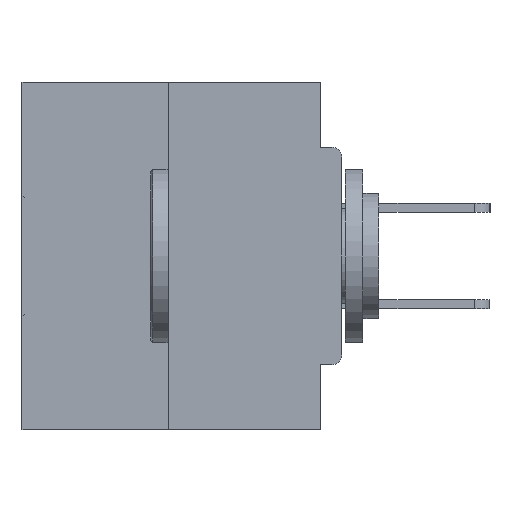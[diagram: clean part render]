
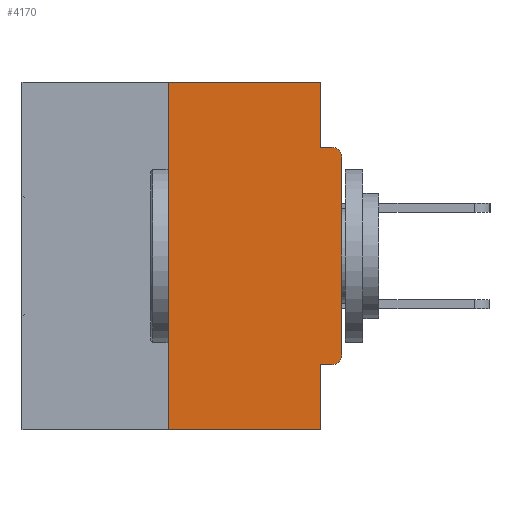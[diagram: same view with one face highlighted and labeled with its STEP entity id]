
A CAD part, left-side view. The second image highlights one B-rep face of the part: STEP entity #4170.
In plain terms, the highlighted planar face has unit normal (-1, 0, 0).
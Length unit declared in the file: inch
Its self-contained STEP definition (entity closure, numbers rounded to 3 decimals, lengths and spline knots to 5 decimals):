
#173 = DIRECTION ( 'NONE',  ( 0., -1., 0. ) ) ;
#609 = VERTEX_POINT ( 'NONE', #1921 ) ;
#1921 = CARTESIAN_POINT ( 'NONE',  ( 0., 0.25, -0.5 ) ) ;
#2100 = EDGE_CURVE ( 'NONE', #4146, #41468, #22063, .T. ) ;
#2630 = CARTESIAN_POINT ( 'NONE',  ( 0., 0.46, 0. ) ) ;
#4146 = VERTEX_POINT ( 'NONE', #24098 ) ;
#4170 = ADVANCED_FACE ( 'NONE', ( #25506 ), #5548, .F. ) ;
#4461 = CIRCLE ( 'NONE', #42442, 0.015 ) ;
#4488 = CARTESIAN_POINT ( 'NONE',  ( 0., 0.015, -0.4065 ) ) ;
#5046 = EDGE_CURVE ( 'NONE', #8070, #19093, #11988, .T. ) ;
#5341 = ORIENTED_EDGE ( 'NONE', *, *, #41812, .T. ) ;
#5405 = CARTESIAN_POINT ( 'NONE',  ( 0., 0.25, 0. ) ) ;
#5548 = PLANE ( 'NONE',  #42159 ) ;
#6233 = CARTESIAN_POINT ( 'NONE',  ( 0., 0.031, -0.5 ) ) ;
#6565 = CARTESIAN_POINT ( 'NONE',  ( 0., 0., -0.4065 ) ) ;
#6663 = VERTEX_POINT ( 'NONE', #5405 ) ;
#7348 = VECTOR ( 'NONE', #12847, 39.37008 ) ;
#8070 = VERTEX_POINT ( 'NONE', #35930 ) ;
#8725 = CARTESIAN_POINT ( 'NONE',  ( 0., 0.25, 0. ) ) ;
#8738 = VECTOR ( 'NONE', #18216, 39.37008 ) ;
#8857 = DIRECTION ( 'NONE',  ( 1., 0., 0. ) ) ;
#9143 = DIRECTION ( 'NONE',  ( 0., 0., -1. ) ) ;
#9898 = CARTESIAN_POINT ( 'NONE',  ( 0., 0., 0. ) ) ;
#10563 = VECTOR ( 'NONE', #173, 39.37008 ) ;
#11882 = LINE ( 'NONE', #35263, #31456 ) ;
#11988 = LINE ( 'NONE', #9898, #38200 ) ;
#12035 = VECTOR ( 'NONE', #12253, 39.37008 ) ;
#12110 = CARTESIAN_POINT ( 'NONE',  ( 0., 0.46, 0. ) ) ;
#12253 = DIRECTION ( 'NONE',  ( 0., -1., 0. ) ) ;
#12656 = VECTOR ( 'NONE', #31747, 39.37008 ) ;
#12847 = DIRECTION ( 'NONE',  ( 0., 1., 0. ) ) ;
#12949 = LINE ( 'NONE', #8725, #41744 ) ;
#14905 = EDGE_CURVE ( 'NONE', #6663, #24951, #20804, .T. ) ;
#15072 = ORIENTED_EDGE ( 'NONE', *, *, #33268, .T. ) ;
#15228 = LINE ( 'NONE', #31597, #12656 ) ;
#17316 = EDGE_CURVE ( 'NONE', #26795, #24085, #11882, .T. ) ;
#17340 = DIRECTION ( 'NONE',  ( -1., 0., 0. ) ) ;
#18037 = DIRECTION ( 'NONE',  ( 0., 0., -1. ) ) ;
#18216 = DIRECTION ( 'NONE',  ( 0., 0., -1. ) ) ;
#19093 = VERTEX_POINT ( 'NONE', #20516 ) ;
#20035 = EDGE_CURVE ( 'NONE', #609, #6663, #12949, .T. ) ;
#20224 = DIRECTION ( 'NONE',  ( 0., 0., 1. ) ) ;
#20516 = CARTESIAN_POINT ( 'NONE',  ( 0., 0., -0.1085 ) ) ;
#20804 = LINE ( 'NONE', #12110, #12035 ) ;
#21762 = AXIS2_PLACEMENT_3D ( 'NONE', #21901, #25218, #18037 ) ;
#21901 = CARTESIAN_POINT ( 'NONE',  ( 0., 0.015, -0.3915 ) ) ;
#22063 = LINE ( 'NONE', #41600, #8738 ) ;
#23034 = CARTESIAN_POINT ( 'NONE',  ( 0., 0.46, -0.5 ) ) ;
#23583 = CIRCLE ( 'NONE', #21762, 0.015 ) ;
#23715 = ORIENTED_EDGE ( 'NONE', *, *, #39460, .F. ) ;
#23766 = ORIENTED_EDGE ( 'NONE', *, *, #20035, .F. ) ;
#24085 = VERTEX_POINT ( 'NONE', #34598 ) ;
#24098 = CARTESIAN_POINT ( 'NONE',  ( 0., 0.031, -0.4065 ) ) ;
#24951 = VERTEX_POINT ( 'NONE', #33543 ) ;
#25218 = DIRECTION ( 'NONE',  ( -1., 0., 0. ) ) ;
#25506 = FACE_OUTER_BOUND ( 'NONE', #36485, .T. ) ;
#25969 = LINE ( 'NONE', #23034, #10563 ) ;
#26795 = VERTEX_POINT ( 'NONE', #27788 ) ;
#27027 = EDGE_CURVE ( 'NONE', #24951, #26795, #15228, .T. ) ;
#27199 = ORIENTED_EDGE ( 'NONE', *, *, #27027, .F. ) ;
#27788 = CARTESIAN_POINT ( 'NONE',  ( 0., 0.031, -0.0935 ) ) ;
#31456 = VECTOR ( 'NONE', #41605, 39.37008 ) ;
#31597 = CARTESIAN_POINT ( 'NONE',  ( 0., 0.031, 0. ) ) ;
#31747 = DIRECTION ( 'NONE',  ( 0., 0., -1. ) ) ;
#31844 = DIRECTION ( 'NONE',  ( 0., 0., 1. ) ) ;
#31912 = ORIENTED_EDGE ( 'NONE', *, *, #5046, .T. ) ;
#32146 = ORIENTED_EDGE ( 'NONE', *, *, #2100, .F. ) ;
#33109 = EDGE_CURVE ( 'NONE', #609, #41468, #25969, .T. ) ;
#33268 = EDGE_CURVE ( 'NONE', #19093, #24085, #4461, .T. ) ;
#33543 = CARTESIAN_POINT ( 'NONE',  ( 0., 0.031, 0. ) ) ;
#34019 = CARTESIAN_POINT ( 'NONE',  ( 0., 0.015, -0.1085 ) ) ;
#34598 = CARTESIAN_POINT ( 'NONE',  ( 0., 0.015, -0.0935 ) ) ;
#35263 = CARTESIAN_POINT ( 'NONE',  ( 0., 0., -0.0935 ) ) ;
#35503 = DIRECTION ( 'NONE',  ( 0., 0., -1. ) ) ;
#35930 = CARTESIAN_POINT ( 'NONE',  ( 0., 0., -0.3915 ) ) ;
#36485 = EDGE_LOOP ( 'NONE', ( #39961, #23766, #39555, #32146, #23715, #5341, #31912, #15072, #40087, #27199 ) ) ;
#38178 = VERTEX_POINT ( 'NONE', #4488 ) ;
#38200 = VECTOR ( 'NONE', #20224, 39.37008 ) ;
#39460 = EDGE_CURVE ( 'NONE', #38178, #4146, #40777, .T. ) ;
#39555 = ORIENTED_EDGE ( 'NONE', *, *, #33109, .T. ) ;
#39961 = ORIENTED_EDGE ( 'NONE', *, *, #14905, .F. ) ;
#40087 = ORIENTED_EDGE ( 'NONE', *, *, #17316, .F. ) ;
#40777 = LINE ( 'NONE', #6565, #7348 ) ;
#41468 = VERTEX_POINT ( 'NONE', #6233 ) ;
#41600 = CARTESIAN_POINT ( 'NONE',  ( 0., 0.031, -0.5 ) ) ;
#41605 = DIRECTION ( 'NONE',  ( 0., -1., 0. ) ) ;
#41744 = VECTOR ( 'NONE', #31844, 39.37008 ) ;
#41812 = EDGE_CURVE ( 'NONE', #38178, #8070, #23583, .T. ) ;
#42159 = AXIS2_PLACEMENT_3D ( 'NONE', #2630, #8857, #35503 ) ;
#42442 = AXIS2_PLACEMENT_3D ( 'NONE', #34019, #17340, #9143 ) ;
